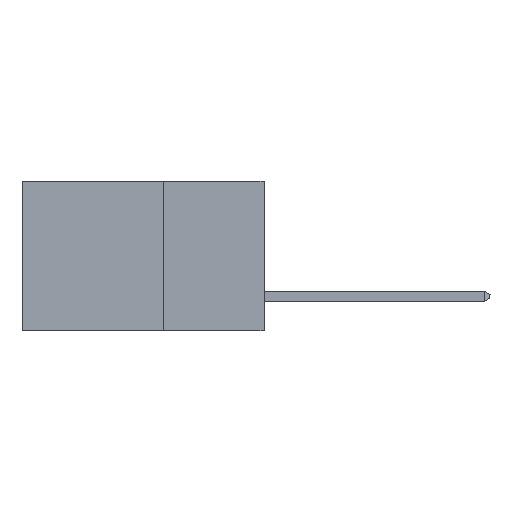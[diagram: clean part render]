
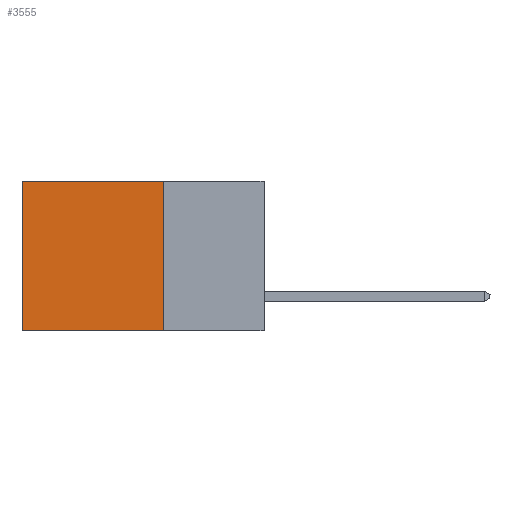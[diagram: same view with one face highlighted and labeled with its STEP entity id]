
A CAD part, left-side view. The second image highlights one B-rep face of the part: STEP entity #3555.
In plain terms, the highlighted planar face has unit normal (-1, 0, 0).
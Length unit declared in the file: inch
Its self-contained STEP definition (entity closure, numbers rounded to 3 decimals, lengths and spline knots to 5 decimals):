
#45 = CARTESIAN_POINT ( 'NONE',  ( 0.2615, 0.6, -0.37 ) ) ;
#309 = VERTEX_POINT ( 'NONE', #2942 ) ;
#667 = ORIENTED_EDGE ( 'NONE', *, *, #669, .T. ) ;
#669 = EDGE_CURVE ( 'NONE', #4848, #749, #10391, .T. ) ;
#679 = EDGE_CURVE ( 'NONE', #10149, #309, #7828, .T. ) ;
#749 = VERTEX_POINT ( 'NONE', #5365 ) ;
#1357 = ORIENTED_EDGE ( 'NONE', *, *, #7406, .F. ) ;
#2648 = DIRECTION ( 'NONE',  ( 0., 0., -1. ) ) ;
#2683 = ORIENTED_EDGE ( 'NONE', *, *, #679, .F. ) ;
#2760 = CARTESIAN_POINT ( 'NONE',  ( 0.2615, 0.25, -0.37 ) ) ;
#2942 = CARTESIAN_POINT ( 'NONE',  ( 0.2615, 0.6, -0.37 ) ) ;
#3330 = PLANE ( 'NONE',  #4725 ) ;
#3555 = ADVANCED_FACE ( 'NONE', ( #11122 ), #3330, .F. ) ;
#3896 = DIRECTION ( 'NONE',  ( 0., 0., -1. ) ) ;
#3949 = LINE ( 'NONE', #4755, #4365 ) ;
#4254 = EDGE_CURVE ( 'NONE', #749, #309, #6990, .T. ) ;
#4365 = VECTOR ( 'NONE', #3896, 39.37008 ) ;
#4725 = AXIS2_PLACEMENT_3D ( 'NONE', #2760, #9749, #2648 ) ;
#4755 = CARTESIAN_POINT ( 'NONE',  ( 0.2615, 0.25, -0.37 ) ) ;
#4848 = VERTEX_POINT ( 'NONE', #9602 ) ;
#5097 = DIRECTION ( 'NONE',  ( 0., 1., 0. ) ) ;
#5365 = CARTESIAN_POINT ( 'NONE',  ( 0.2615, 0.6, 0. ) ) ;
#6990 = LINE ( 'NONE', #45, #8679 ) ;
#7406 = EDGE_CURVE ( 'NONE', #4848, #10149, #3949, .T. ) ;
#7506 = VECTOR ( 'NONE', #5097, 39.37008 ) ;
#7763 = CARTESIAN_POINT ( 'NONE',  ( 0.2615, 0.25, -0.37 ) ) ;
#7828 = LINE ( 'NONE', #11241, #8954 ) ;
#8198 = EDGE_LOOP ( 'NONE', ( #8248, #2683, #1357, #667 ) ) ;
#8248 = ORIENTED_EDGE ( 'NONE', *, *, #4254, .T. ) ;
#8508 = DIRECTION ( 'NONE',  ( 0., 1., 0. ) ) ;
#8679 = VECTOR ( 'NONE', #11076, 39.37008 ) ;
#8954 = VECTOR ( 'NONE', #8508, 39.37008 ) ;
#9499 = CARTESIAN_POINT ( 'NONE',  ( 0.2615, 0.25, 0. ) ) ;
#9602 = CARTESIAN_POINT ( 'NONE',  ( 0.2615, 0.25, 0. ) ) ;
#9749 = DIRECTION ( 'NONE',  ( 1., 0., 0. ) ) ;
#10149 = VERTEX_POINT ( 'NONE', #7763 ) ;
#10391 = LINE ( 'NONE', #9499, #7506 ) ;
#11076 = DIRECTION ( 'NONE',  ( 0., 0., -1. ) ) ;
#11122 = FACE_OUTER_BOUND ( 'NONE', #8198, .T. ) ;
#11241 = CARTESIAN_POINT ( 'NONE',  ( 0.2615, 0.25, -0.37 ) ) ;
